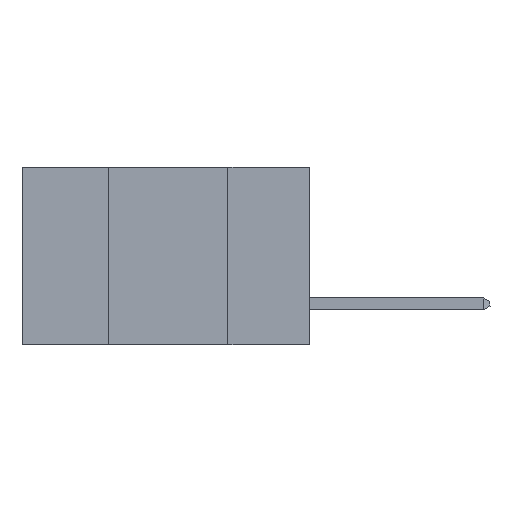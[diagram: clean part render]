
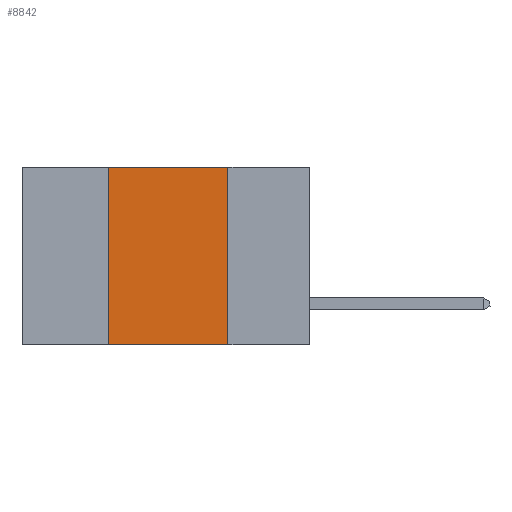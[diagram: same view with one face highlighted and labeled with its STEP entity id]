
A CAD part, left-side view. The second image highlights one B-rep face of the part: STEP entity #8842.
In plain terms, the highlighted planar face has unit normal (-1, 0, 0).
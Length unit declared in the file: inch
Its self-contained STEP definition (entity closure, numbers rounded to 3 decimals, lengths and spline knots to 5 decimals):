
#167 = CARTESIAN_POINT ( 'NONE',  ( 0., 0.42, 0. ) ) ;
#758 = VERTEX_POINT ( 'NONE', #2237 ) ;
#799 = VERTEX_POINT ( 'NONE', #7064 ) ;
#1237 = EDGE_LOOP ( 'NONE', ( #4993, #5047, #5152, #5348 ) ) ;
#1279 = DIRECTION ( 'NONE',  ( 0., 0., 1. ) ) ;
#1410 = LINE ( 'NONE', #4159, #6434 ) ;
#1459 = PLANE ( 'NONE',  #4473 ) ;
#1783 = EDGE_CURVE ( 'NONE', #758, #799, #9899, .T. ) ;
#1942 = EDGE_CURVE ( 'NONE', #799, #11398, #1410, .T. ) ;
#2022 = CARTESIAN_POINT ( 'NONE',  ( 0., 0.6, 0. ) ) ;
#2237 = CARTESIAN_POINT ( 'NONE',  ( 0., 0.42, 0. ) ) ;
#2609 = CARTESIAN_POINT ( 'NONE',  ( 0., 0.6, -0.37 ) ) ;
#3070 = DIRECTION ( 'NONE',  ( 0., -1., 0. ) ) ;
#3160 = VERTEX_POINT ( 'NONE', #7534 ) ;
#3254 = DIRECTION ( 'NONE',  ( 0., 0., -1. ) ) ;
#3512 = DIRECTION ( 'NONE',  ( 1., 0., 0. ) ) ;
#4159 = CARTESIAN_POINT ( 'NONE',  ( 0., 0.17, 0. ) ) ;
#4473 = AXIS2_PLACEMENT_3D ( 'NONE', #6176, #3512, #9743 ) ;
#4520 = VECTOR ( 'NONE', #1279, 39.37008 ) ;
#4596 = CARTESIAN_POINT ( 'NONE',  ( 0., 0.17, -0.37 ) ) ;
#4805 = LINE ( 'NONE', #167, #4520 ) ;
#4993 = ORIENTED_EDGE ( 'NONE', *, *, #1942, .F. ) ;
#5047 = ORIENTED_EDGE ( 'NONE', *, *, #1783, .F. ) ;
#5152 = ORIENTED_EDGE ( 'NONE', *, *, #11186, .F. ) ;
#5348 = ORIENTED_EDGE ( 'NONE', *, *, #7783, .T. ) ;
#5710 = VECTOR ( 'NONE', #8069, 39.37008 ) ;
#6176 = CARTESIAN_POINT ( 'NONE',  ( 0., 0.6, 0. ) ) ;
#6434 = VECTOR ( 'NONE', #3254, 39.37008 ) ;
#7064 = CARTESIAN_POINT ( 'NONE',  ( 0., 0.17, 0. ) ) ;
#7534 = CARTESIAN_POINT ( 'NONE',  ( 0., 0.42, -0.37 ) ) ;
#7612 = VECTOR ( 'NONE', #3070, 39.37008 ) ;
#7783 = EDGE_CURVE ( 'NONE', #3160, #11398, #10395, .T. ) ;
#8069 = DIRECTION ( 'NONE',  ( 0., -1., 0. ) ) ;
#8842 = ADVANCED_FACE ( 'NONE', ( #9972 ), #1459, .F. ) ;
#9743 = DIRECTION ( 'NONE',  ( 0., 0., -1. ) ) ;
#9899 = LINE ( 'NONE', #2022, #7612 ) ;
#9972 = FACE_OUTER_BOUND ( 'NONE', #1237, .T. ) ;
#10395 = LINE ( 'NONE', #2609, #5710 ) ;
#11186 = EDGE_CURVE ( 'NONE', #3160, #758, #4805, .T. ) ;
#11398 = VERTEX_POINT ( 'NONE', #4596 ) ;
